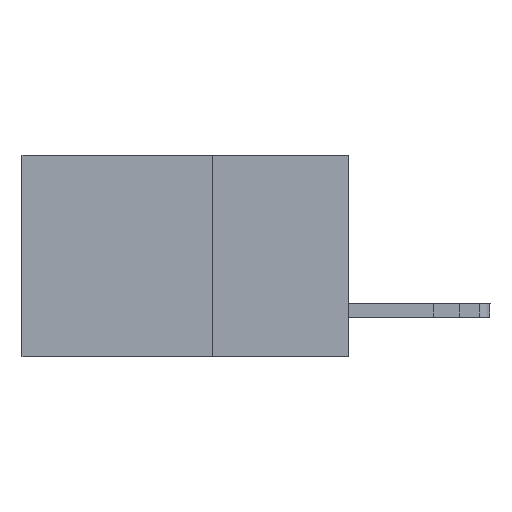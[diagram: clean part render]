
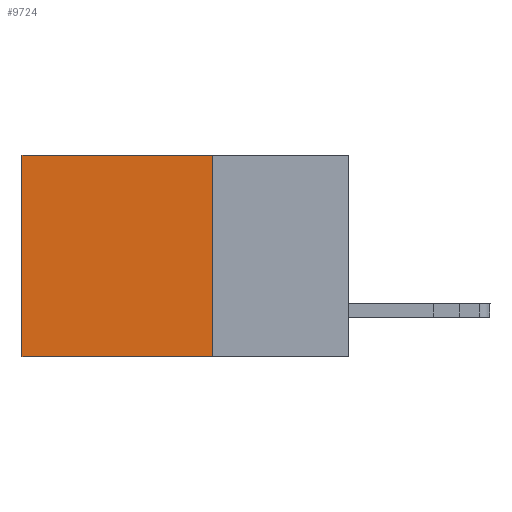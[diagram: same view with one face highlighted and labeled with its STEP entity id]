
A CAD part, left-side view. The second image highlights one B-rep face of the part: STEP entity #9724.
In plain terms, the highlighted planar face has unit normal (-1, 0, 0).
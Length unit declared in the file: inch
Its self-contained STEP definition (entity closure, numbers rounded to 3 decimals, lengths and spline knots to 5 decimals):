
#118 = EDGE_CURVE ( 'NONE', #14597, #206, #11994, .T. ) ;
#206 = VERTEX_POINT ( 'NONE', #6663 ) ;
#904 = CARTESIAN_POINT ( 'NONE',  ( 0.2615, 0.25, -0.37 ) ) ;
#2856 = AXIS2_PLACEMENT_3D ( 'NONE', #3969, #6589, #13960 ) ;
#2983 = DIRECTION ( 'NONE',  ( 0., 1., 0. ) ) ;
#3348 = CARTESIAN_POINT ( 'NONE',  ( 0.2615, 0.25, 0. ) ) ;
#3600 = LINE ( 'NONE', #904, #13864 ) ;
#3969 = CARTESIAN_POINT ( 'NONE',  ( 0.2615, 0.25, -0.37 ) ) ;
#4248 = CARTESIAN_POINT ( 'NONE',  ( 0.2615, 0.25, -0.37 ) ) ;
#4998 = ORIENTED_EDGE ( 'NONE', *, *, #118, .T. ) ;
#5292 = EDGE_LOOP ( 'NONE', ( #12971, #10148, #9767, #4998 ) ) ;
#5819 = VERTEX_POINT ( 'NONE', #11900 ) ;
#6068 = EDGE_CURVE ( 'NONE', #14597, #5819, #3600, .T. ) ;
#6589 = DIRECTION ( 'NONE',  ( 1., 0., 0. ) ) ;
#6663 = CARTESIAN_POINT ( 'NONE',  ( 0.2615, 0.6, 0. ) ) ;
#6880 = LINE ( 'NONE', #14886, #13744 ) ;
#7868 = PLANE ( 'NONE',  #2856 ) ;
#8135 = VERTEX_POINT ( 'NONE', #8969 ) ;
#8407 = DIRECTION ( 'NONE',  ( 0., 0., -1. ) ) ;
#8969 = CARTESIAN_POINT ( 'NONE',  ( 0.2615, 0.6, -0.37 ) ) ;
#9724 = ADVANCED_FACE ( 'NONE', ( #15619 ), #7868, .F. ) ;
#9767 = ORIENTED_EDGE ( 'NONE', *, *, #6068, .F. ) ;
#10148 = ORIENTED_EDGE ( 'NONE', *, *, #12280, .F. ) ;
#10196 = VECTOR ( 'NONE', #2983, 39.37008 ) ;
#10569 = CARTESIAN_POINT ( 'NONE',  ( 0.2615, 0.25, 0. ) ) ;
#10815 = DIRECTION ( 'NONE',  ( 0., 1., 0. ) ) ;
#10851 = LINE ( 'NONE', #4248, #10196 ) ;
#11304 = DIRECTION ( 'NONE',  ( 0., 0., -1. ) ) ;
#11900 = CARTESIAN_POINT ( 'NONE',  ( 0.2615, 0.25, -0.37 ) ) ;
#11994 = LINE ( 'NONE', #10569, #15682 ) ;
#12280 = EDGE_CURVE ( 'NONE', #5819, #8135, #10851, .T. ) ;
#12971 = ORIENTED_EDGE ( 'NONE', *, *, #14981, .T. ) ;
#13744 = VECTOR ( 'NONE', #8407, 39.37008 ) ;
#13864 = VECTOR ( 'NONE', #11304, 39.37008 ) ;
#13960 = DIRECTION ( 'NONE',  ( 0., 0., -1. ) ) ;
#14597 = VERTEX_POINT ( 'NONE', #3348 ) ;
#14886 = CARTESIAN_POINT ( 'NONE',  ( 0.2615, 0.6, -0.37 ) ) ;
#14981 = EDGE_CURVE ( 'NONE', #206, #8135, #6880, .T. ) ;
#15619 = FACE_OUTER_BOUND ( 'NONE', #5292, .T. ) ;
#15682 = VECTOR ( 'NONE', #10815, 39.37008 ) ;
